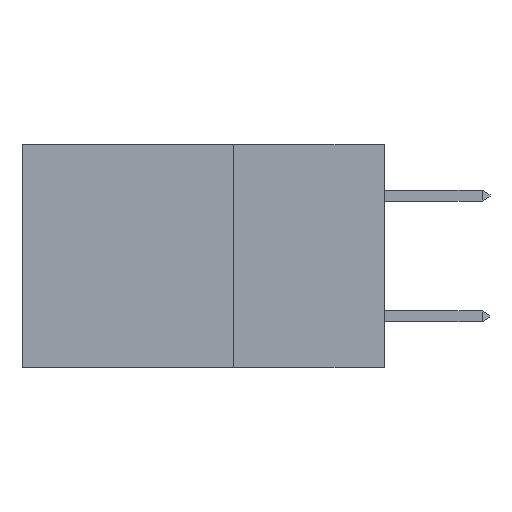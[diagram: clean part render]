
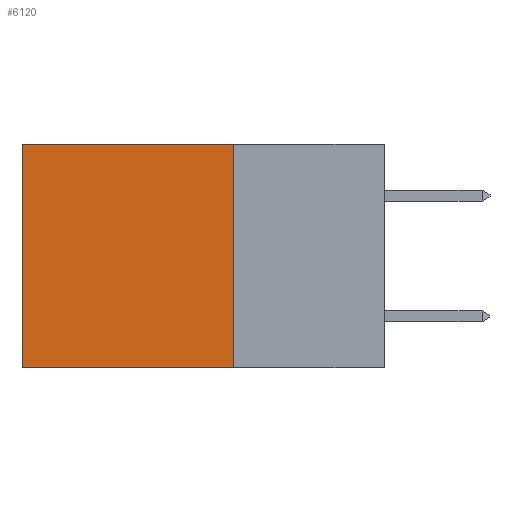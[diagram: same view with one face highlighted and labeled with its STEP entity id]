
A CAD part, left-side view. The second image highlights one B-rep face of the part: STEP entity #6120.
In plain terms, the highlighted planar face has unit normal (-1, 0, 0).
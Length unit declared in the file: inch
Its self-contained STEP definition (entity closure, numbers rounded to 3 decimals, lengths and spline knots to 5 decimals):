
#155 = ORIENTED_EDGE ( 'NONE', *, *, #3072, .T. ) ;
#224 = VERTEX_POINT ( 'NONE', #6460 ) ;
#701 = ORIENTED_EDGE ( 'NONE', *, *, #4817, .F. ) ;
#714 = ORIENTED_EDGE ( 'NONE', *, *, #7660, .F. ) ;
#1389 = ORIENTED_EDGE ( 'NONE', *, *, #8351, .T. ) ;
#1606 = DIRECTION ( 'NONE',  ( 0., 0., -1. ) ) ;
#1633 = DIRECTION ( 'NONE',  ( 1., 0., 0. ) ) ;
#1687 = CARTESIAN_POINT ( 'NONE',  ( 0.2875, 0.6, -0.37 ) ) ;
#1754 = CARTESIAN_POINT ( 'NONE',  ( 0.2875, 0.25, 0. ) ) ;
#1773 = CARTESIAN_POINT ( 'NONE',  ( 0.2875, 0.25, -0.37 ) ) ;
#1778 = PLANE ( 'NONE',  #2182 ) ;
#2182 = AXIS2_PLACEMENT_3D ( 'NONE', #1754, #1633, #1606 ) ;
#2427 = VECTOR ( 'NONE', #4123, 39.37008 ) ;
#2430 = DIRECTION ( 'NONE',  ( 0., 1., 0. ) ) ;
#2886 = VERTEX_POINT ( 'NONE', #1687 ) ;
#3072 = EDGE_CURVE ( 'NONE', #3111, #2886, #8628, .T. ) ;
#3111 = VERTEX_POINT ( 'NONE', #5267 ) ;
#3875 = CARTESIAN_POINT ( 'NONE',  ( 0.2875, 0.25, 0. ) ) ;
#4123 = DIRECTION ( 'NONE',  ( 0., 1., 0. ) ) ;
#4408 = VERTEX_POINT ( 'NONE', #1773 ) ;
#4504 = CARTESIAN_POINT ( 'NONE',  ( 0.2875, 0.25, -0.37 ) ) ;
#4744 = VECTOR ( 'NONE', #6090, 39.37008 ) ;
#4817 = EDGE_CURVE ( 'NONE', #4408, #2886, #7720, .T. ) ;
#5267 = CARTESIAN_POINT ( 'NONE',  ( 0.2875, 0.6, 0. ) ) ;
#6090 = DIRECTION ( 'NONE',  ( 0., 0., -1. ) ) ;
#6101 = EDGE_LOOP ( 'NONE', ( #155, #701, #714, #1389 ) ) ;
#6120 = ADVANCED_FACE ( 'NONE', ( #8411 ), #1778, .F. ) ;
#6460 = CARTESIAN_POINT ( 'NONE',  ( 0.2875, 0.25, 0. ) ) ;
#6716 = CARTESIAN_POINT ( 'NONE',  ( 0.2875, 0.25, 0. ) ) ;
#6806 = VECTOR ( 'NONE', #2430, 39.37008 ) ;
#6877 = DIRECTION ( 'NONE',  ( 0., 0., -1. ) ) ;
#7086 = VECTOR ( 'NONE', #6877, 39.37008 ) ;
#7240 = CARTESIAN_POINT ( 'NONE',  ( 0.2875, 0.6, 0. ) ) ;
#7660 = EDGE_CURVE ( 'NONE', #224, #4408, #8486, .T. ) ;
#7720 = LINE ( 'NONE', #4504, #2427 ) ;
#8351 = EDGE_CURVE ( 'NONE', #224, #3111, #8386, .T. ) ;
#8386 = LINE ( 'NONE', #3875, #6806 ) ;
#8411 = FACE_OUTER_BOUND ( 'NONE', #6101, .T. ) ;
#8486 = LINE ( 'NONE', #6716, #4744 ) ;
#8628 = LINE ( 'NONE', #7240, #7086 ) ;
